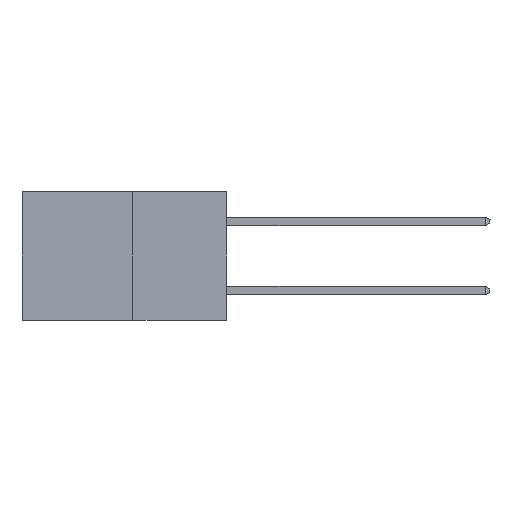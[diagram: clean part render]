
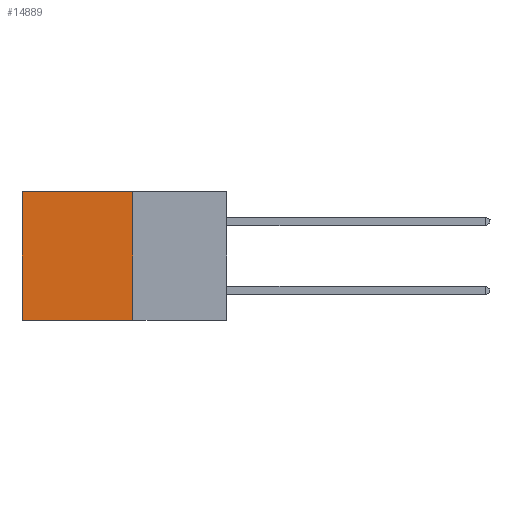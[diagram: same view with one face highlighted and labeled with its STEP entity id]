
A CAD part, left-side view. The second image highlights one B-rep face of the part: STEP entity #14889.
In plain terms, the highlighted planar face has unit normal (-1, 0, 0).
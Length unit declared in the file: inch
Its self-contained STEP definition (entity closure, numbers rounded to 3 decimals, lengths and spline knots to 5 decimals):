
#841 = ORIENTED_EDGE ( 'NONE', *, *, #5808, .F. ) ;
#1009 = ORIENTED_EDGE ( 'NONE', *, *, #2795, .T. ) ;
#1098 = FACE_OUTER_BOUND ( 'NONE', #4183, .T. ) ;
#1493 = CARTESIAN_POINT ( 'NONE',  ( 0.277, 0.27, -0.37 ) ) ;
#2451 = VECTOR ( 'NONE', #13523, 39.37008 ) ;
#2519 = VERTEX_POINT ( 'NONE', #15566 ) ;
#2795 = EDGE_CURVE ( 'NONE', #4249, #2519, #15200, .T. ) ;
#2811 = LINE ( 'NONE', #12327, #2451 ) ;
#4183 = EDGE_LOOP ( 'NONE', ( #1009, #841, #8289, #10097 ) ) ;
#4249 = VERTEX_POINT ( 'NONE', #4634 ) ;
#4634 = CARTESIAN_POINT ( 'NONE',  ( 0.277, 0.59, 0. ) ) ;
#5808 = EDGE_CURVE ( 'NONE', #15058, #2519, #11947, .T. ) ;
#5985 = PLANE ( 'NONE',  #13529 ) ;
#6225 = DIRECTION ( 'NONE',  ( 0., 0., -1. ) ) ;
#6429 = LINE ( 'NONE', #12627, #15236 ) ;
#6712 = CARTESIAN_POINT ( 'NONE',  ( 0.277, 0.27, -0.37 ) ) ;
#7216 = CARTESIAN_POINT ( 'NONE',  ( 0.277, 0.27, -0.37 ) ) ;
#8243 = CARTESIAN_POINT ( 'NONE',  ( 0.277, 0.27, 0. ) ) ;
#8289 = ORIENTED_EDGE ( 'NONE', *, *, #14363, .F. ) ;
#8440 = DIRECTION ( 'NONE',  ( 0., 0., -1. ) ) ;
#8590 = VERTEX_POINT ( 'NONE', #8243 ) ;
#8714 = VECTOR ( 'NONE', #15099, 39.37008 ) ;
#10097 = ORIENTED_EDGE ( 'NONE', *, *, #11881, .T. ) ;
#11881 = EDGE_CURVE ( 'NONE', #8590, #4249, #6429, .T. ) ;
#11947 = LINE ( 'NONE', #6712, #8714 ) ;
#12123 = VECTOR ( 'NONE', #6225, 39.37008 ) ;
#12327 = CARTESIAN_POINT ( 'NONE',  ( 0.277, 0.27, -0.37 ) ) ;
#12627 = CARTESIAN_POINT ( 'NONE',  ( 0.277, 0.27, 0. ) ) ;
#13523 = DIRECTION ( 'NONE',  ( 0., 0., -1. ) ) ;
#13529 = AXIS2_PLACEMENT_3D ( 'NONE', #7216, #15531, #8440 ) ;
#13828 = DIRECTION ( 'NONE',  ( 0., 1., 0. ) ) ;
#14363 = EDGE_CURVE ( 'NONE', #8590, #15058, #2811, .T. ) ;
#14889 = ADVANCED_FACE ( 'NONE', ( #1098 ), #5985, .F. ) ;
#15058 = VERTEX_POINT ( 'NONE', #1493 ) ;
#15099 = DIRECTION ( 'NONE',  ( 0., 1., 0. ) ) ;
#15200 = LINE ( 'NONE', #15499, #12123 ) ;
#15236 = VECTOR ( 'NONE', #13828, 39.37008 ) ;
#15499 = CARTESIAN_POINT ( 'NONE',  ( 0.277, 0.59, -0.37 ) ) ;
#15531 = DIRECTION ( 'NONE',  ( 1., 0., 0. ) ) ;
#15566 = CARTESIAN_POINT ( 'NONE',  ( 0.277, 0.59, -0.37 ) ) ;
